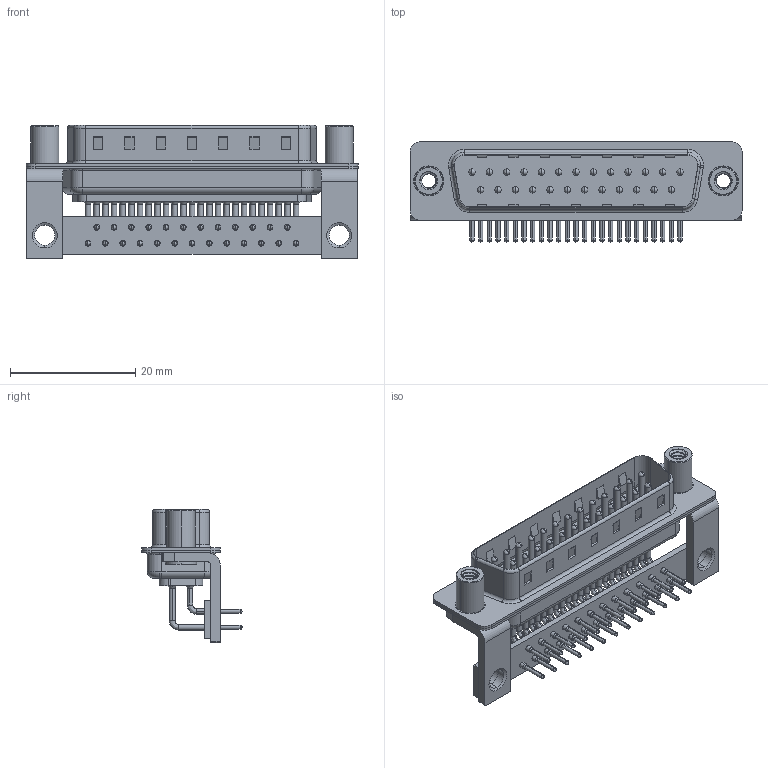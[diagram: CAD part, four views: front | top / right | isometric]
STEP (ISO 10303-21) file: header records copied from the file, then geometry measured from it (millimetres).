
FILE_DESCRIPTION (( 'STEP AP203' ), '1' );
FILE_NAME ('629-M25-640-BN6.STEP', '2018-09-25T20:16:05', ( '' ), ( '' ), 'SwSTEP 2.0', 'SolidWorks 2016', '' );
FILE_SCHEMA (( 'CONFIG_CONTROL_DESIGN' ));
Length unit declared in the file: millimetre
Products named in the file (9): 629M Stabilizer Board_25 Contacts; 629-M25-640-BN6; 629M Housing_25 Contacts; 629M Shell Front_25 Contacts; 629M Shell Rear_25 Contacts; 629M Contact Row 1; 629M Contact Row 2; 629M Stabilizer Bracket; 629M 4-40 Threaded Standoff
Assembly tree (33 placements, depth 2):
  629-M25-640-BN6
    629M Housing_25 Contacts
    629M Shell Front_25 Contacts
    629M Shell Rear_25 Contacts
    629M Contact Row 1  x13
    629M Contact Row 2  x12
    629M Stabilizer Bracket  x2
    629M 4-40 Threaded Standoff  x2
    629M Stabilizer Board_25 Contacts
Bounding box: 53.05 x 16 x 21.3 mm (x, y, z)
Volume: 3591.7 mm3; surface area: 9450.5 mm2
Topology: 33 solids, 33 shells, 3276 faces, 9153 edges, 5956 vertices
Faces by surface type: plane 1799, cylinder 1151, bspline 156, cone 114, torus 56
Entity records: 30048 total; most frequent: CARTESIAN_POINT 6656, DIRECTION 4747, ORIENTED_EDGE 4402, EDGE_CURVE 2201, AXIS2_PLACEMENT_3D 1754, VERTEX_POINT 1429, LINE 1239, VECTOR 1239
